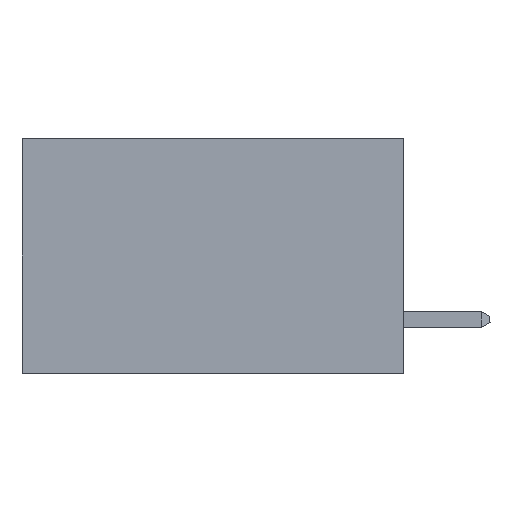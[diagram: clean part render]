
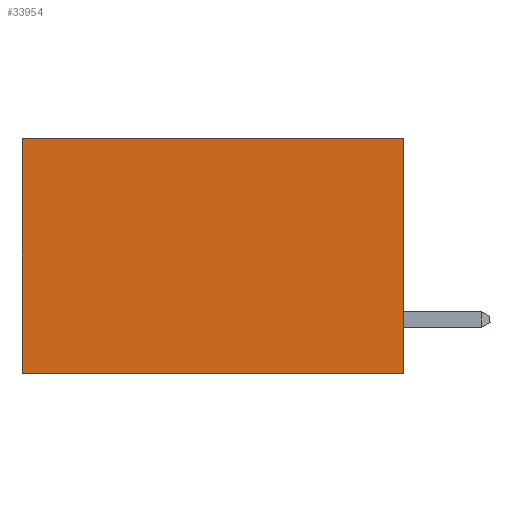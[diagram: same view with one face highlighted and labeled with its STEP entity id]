
A CAD part, left-side view. The second image highlights one B-rep face of the part: STEP entity #33954.
In plain terms, the highlighted planar face has unit normal (-1, 0, 0).
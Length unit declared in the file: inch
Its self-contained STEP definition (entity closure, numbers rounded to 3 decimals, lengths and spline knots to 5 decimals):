
#220 = VECTOR ( 'NONE', #15634, 39.37008 ) ;
#1411 = ORIENTED_EDGE ( 'NONE', *, *, #32584, .T. ) ;
#1473 = EDGE_CURVE ( 'NONE', #35559, #21420, #30484, .T. ) ;
#3271 = LINE ( 'NONE', #14777, #32421 ) ;
#4273 = VERTEX_POINT ( 'NONE', #20370 ) ;
#5141 = CARTESIAN_POINT ( 'NONE',  ( 0.2875, 0., -0.37 ) ) ;
#5760 = CARTESIAN_POINT ( 'NONE',  ( 0.2875, 0., 0. ) ) ;
#6534 = ORIENTED_EDGE ( 'NONE', *, *, #35312, .T. ) ;
#8127 = VECTOR ( 'NONE', #28131, 39.37008 ) ;
#8219 = DIRECTION ( 'NONE',  ( 0., 0., -1. ) ) ;
#8478 = CARTESIAN_POINT ( 'NONE',  ( 0.2875, 0., 0. ) ) ;
#10849 = ORIENTED_EDGE ( 'NONE', *, *, #21559, .F. ) ;
#14777 = CARTESIAN_POINT ( 'NONE',  ( 0.2875, 0.6, 0. ) ) ;
#15177 = PLANE ( 'NONE',  #35930 ) ;
#15326 = DIRECTION ( 'NONE',  ( 0., 0., -1. ) ) ;
#15634 = DIRECTION ( 'NONE',  ( 0., 0., -1. ) ) ;
#15784 = DIRECTION ( 'NONE',  ( 0., 1., 0. ) ) ;
#18054 = VECTOR ( 'NONE', #15784, 39.37008 ) ;
#20370 = CARTESIAN_POINT ( 'NONE',  ( 0.2875, 0.6, 0. ) ) ;
#21420 = VERTEX_POINT ( 'NONE', #41971 ) ;
#21559 = EDGE_CURVE ( 'NONE', #39456, #35559, #23589, .T. ) ;
#21837 = DIRECTION ( 'NONE',  ( 1., 0., 0. ) ) ;
#23589 = LINE ( 'NONE', #29132, #220 ) ;
#25727 = ORIENTED_EDGE ( 'NONE', *, *, #1473, .F. ) ;
#28131 = DIRECTION ( 'NONE',  ( 0., 1., 0. ) ) ;
#29132 = CARTESIAN_POINT ( 'NONE',  ( 0.2875, 0., 0. ) ) ;
#30484 = LINE ( 'NONE', #5141, #8127 ) ;
#32421 = VECTOR ( 'NONE', #8219, 39.37008 ) ;
#32584 = EDGE_CURVE ( 'NONE', #4273, #21420, #3271, .T. ) ;
#33954 = ADVANCED_FACE ( 'NONE', ( #34816 ), #15177, .F. ) ;
#34816 = FACE_OUTER_BOUND ( 'NONE', #36269, .T. ) ;
#35312 = EDGE_CURVE ( 'NONE', #39456, #4273, #35811, .T. ) ;
#35559 = VERTEX_POINT ( 'NONE', #36902 ) ;
#35811 = LINE ( 'NONE', #5760, #18054 ) ;
#35930 = AXIS2_PLACEMENT_3D ( 'NONE', #8478, #21837, #15326 ) ;
#36269 = EDGE_LOOP ( 'NONE', ( #1411, #25727, #10849, #6534 ) ) ;
#36902 = CARTESIAN_POINT ( 'NONE',  ( 0.2875, 0., -0.37 ) ) ;
#37789 = CARTESIAN_POINT ( 'NONE',  ( 0.2875, 0., 0. ) ) ;
#39456 = VERTEX_POINT ( 'NONE', #37789 ) ;
#41971 = CARTESIAN_POINT ( 'NONE',  ( 0.2875, 0.6, -0.37 ) ) ;
